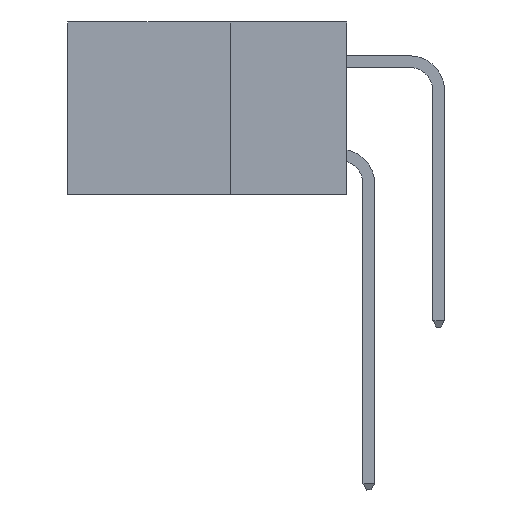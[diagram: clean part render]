
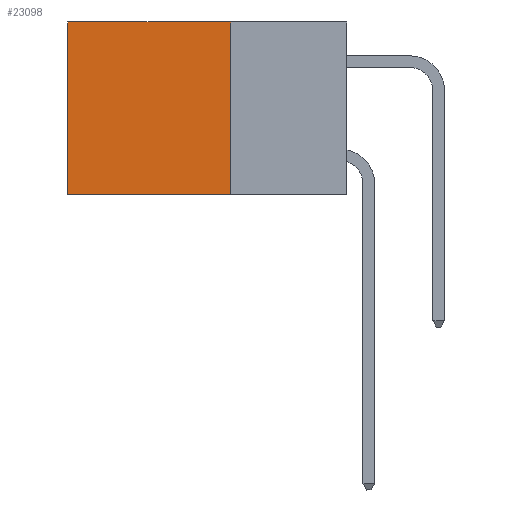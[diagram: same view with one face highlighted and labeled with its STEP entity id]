
A CAD part, left-side view. The second image highlights one B-rep face of the part: STEP entity #23098.
In plain terms, the highlighted planar face has unit normal (-1, 0, 0).
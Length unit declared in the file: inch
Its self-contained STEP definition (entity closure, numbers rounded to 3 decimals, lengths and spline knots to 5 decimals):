
#525 = VERTEX_POINT ( 'NONE', #1977 ) ;
#587 = ORIENTED_EDGE ( 'NONE', *, *, #20124, .T. ) ;
#1977 = CARTESIAN_POINT ( 'NONE',  ( 0.2875, 0.25, 0. ) ) ;
#3826 = CARTESIAN_POINT ( 'NONE',  ( 0.2875, 0.25, 0. ) ) ;
#7956 = DIRECTION ( 'NONE',  ( 0., 0., -1. ) ) ;
#9047 = DIRECTION ( 'NONE',  ( 0., 0., -1. ) ) ;
#9671 = ORIENTED_EDGE ( 'NONE', *, *, #41647, .F. ) ;
#10277 = LINE ( 'NONE', #3826, #17262 ) ;
#14724 = DIRECTION ( 'NONE',  ( 1., 0., 0. ) ) ;
#15236 = LINE ( 'NONE', #40399, #28073 ) ;
#16509 = VECTOR ( 'NONE', #9047, 39.37008 ) ;
#17262 = VECTOR ( 'NONE', #21029, 39.37008 ) ;
#18404 = LINE ( 'NONE', #30823, #24819 ) ;
#18539 = CARTESIAN_POINT ( 'NONE',  ( 0.2875, 0.6, -0.37 ) ) ;
#18739 = EDGE_CURVE ( 'NONE', #525, #34312, #15236, .T. ) ;
#20124 = EDGE_CURVE ( 'NONE', #525, #23017, #10277, .T. ) ;
#21029 = DIRECTION ( 'NONE',  ( 0., 1., 0. ) ) ;
#22449 = ORIENTED_EDGE ( 'NONE', *, *, #18739, .F. ) ;
#23017 = VERTEX_POINT ( 'NONE', #38340 ) ;
#23098 = ADVANCED_FACE ( 'NONE', ( #27681 ), #38788, .F. ) ;
#23388 = CARTESIAN_POINT ( 'NONE',  ( 0.2875, 0.25, -0.37 ) ) ;
#24819 = VECTOR ( 'NONE', #25119, 39.37008 ) ;
#25119 = DIRECTION ( 'NONE',  ( 0., 1., 0. ) ) ;
#25660 = ORIENTED_EDGE ( 'NONE', *, *, #34220, .T. ) ;
#25802 = CARTESIAN_POINT ( 'NONE',  ( 0.2875, 0.6, 0. ) ) ;
#26079 = EDGE_LOOP ( 'NONE', ( #25660, #9671, #22449, #587 ) ) ;
#27252 = DIRECTION ( 'NONE',  ( 0., 0., -1. ) ) ;
#27681 = FACE_OUTER_BOUND ( 'NONE', #26079, .T. ) ;
#28073 = VECTOR ( 'NONE', #27252, 39.37008 ) ;
#30823 = CARTESIAN_POINT ( 'NONE',  ( 0.2875, 0.25, -0.37 ) ) ;
#30950 = LINE ( 'NONE', #25802, #16509 ) ;
#31770 = CARTESIAN_POINT ( 'NONE',  ( 0.2875, 0.25, 0. ) ) ;
#34220 = EDGE_CURVE ( 'NONE', #23017, #39973, #30950, .T. ) ;
#34312 = VERTEX_POINT ( 'NONE', #23388 ) ;
#37435 = AXIS2_PLACEMENT_3D ( 'NONE', #31770, #14724, #7956 ) ;
#38340 = CARTESIAN_POINT ( 'NONE',  ( 0.2875, 0.6, 0. ) ) ;
#38788 = PLANE ( 'NONE',  #37435 ) ;
#39973 = VERTEX_POINT ( 'NONE', #18539 ) ;
#40399 = CARTESIAN_POINT ( 'NONE',  ( 0.2875, 0.25, 0. ) ) ;
#41647 = EDGE_CURVE ( 'NONE', #34312, #39973, #18404, .T. ) ;
